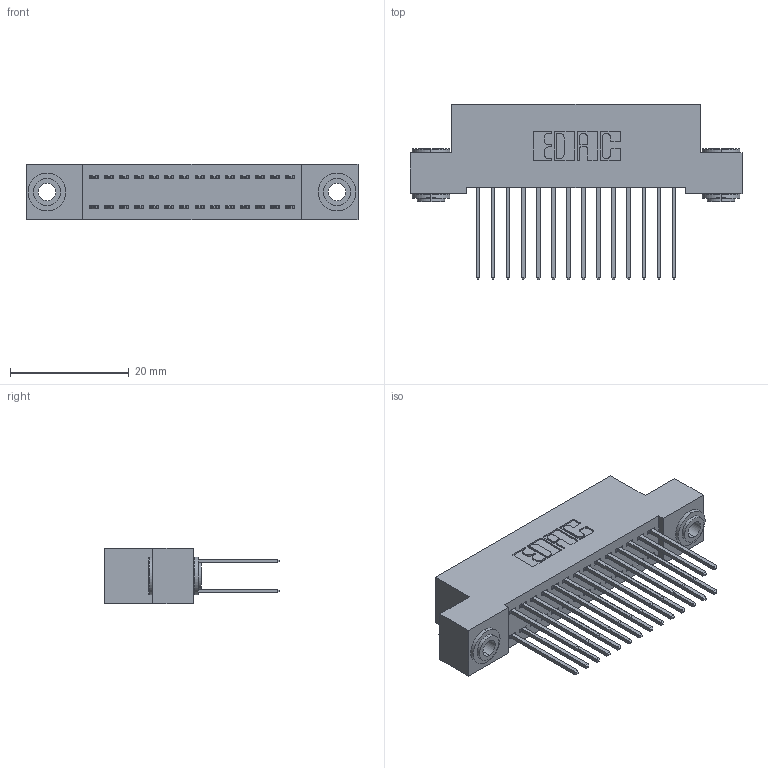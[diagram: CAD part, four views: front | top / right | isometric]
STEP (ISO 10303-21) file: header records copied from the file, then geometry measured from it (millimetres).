
FILE_DESCRIPTION (( 'STEP AP203' ), '1' );
FILE_NAME ('392-028-540-203.STEP', '2019-10-07T12:21:24', ( '' ), ( '' ), 'SwSTEP 2.0', 'SolidWorks 2016', '' );
FILE_SCHEMA (( 'CONFIG_CONTROL_DESIGN' ));
Length unit declared in the file: inch
Products named in the file (4): 342 Part_.156 TH; 345-292-001_345-293-140; 342-250-002_345-250-002-102; 392-028-540-203
Assembly tree (31 placements, depth 2):
  392-028-540-203
    342 Part_.156 TH
    345-292-001_345-293-140  x28
    342-250-002_345-250-002-102  x2
Bounding box: 55.88 x 29.47 x 9.4 mm (x, y, z)
Volume: 5017.2 mm3; surface area: 8162.8 mm2
Topology: 31 solids, 31 shells, 1604 faces, 4715 edges, 3102 vertices
Faces by surface type: plane 1084, cylinder 512, cone 8
Entity records: 13164 total; most frequent: CARTESIAN_POINT 2189, ORIENTED_EDGE 2118, DIRECTION 1953, EDGE_CURVE 1059, VECTOR 907, LINE 907, VERTEX_POINT 702, AXIS2_PLACEMENT_3D 523
